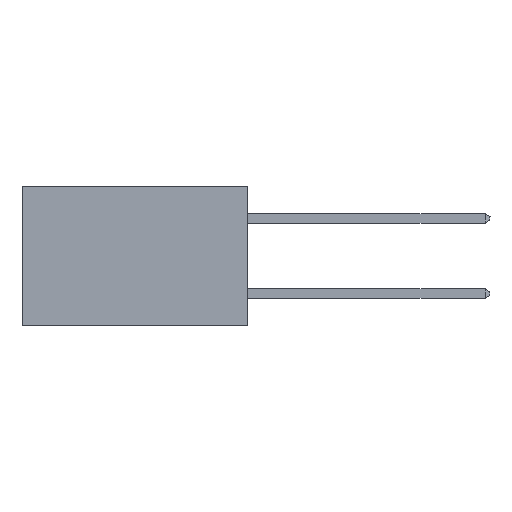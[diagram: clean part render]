
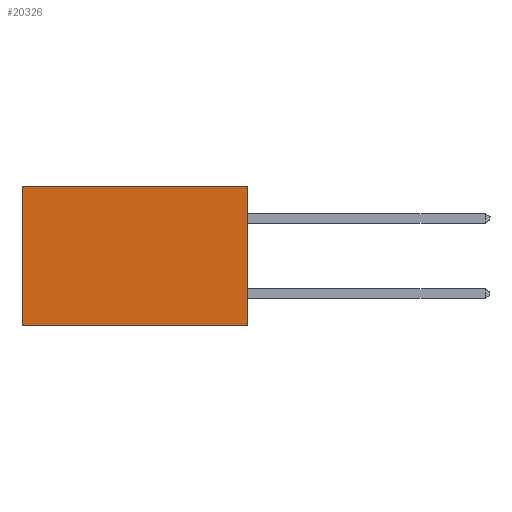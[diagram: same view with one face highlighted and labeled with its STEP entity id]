
A CAD part, left-side view. The second image highlights one B-rep face of the part: STEP entity #20326.
In plain terms, the highlighted planar face has unit normal (-1, 0, 0).
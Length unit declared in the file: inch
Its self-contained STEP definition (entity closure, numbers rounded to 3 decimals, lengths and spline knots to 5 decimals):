
#778 = LINE ( 'NONE', #7036, #1681 ) ;
#897 = FACE_OUTER_BOUND ( 'NONE', #9517, .T. ) ;
#1343 = LINE ( 'NONE', #14374, #9402 ) ;
#1681 = VECTOR ( 'NONE', #18409, 39.37008 ) ;
#2410 = VERTEX_POINT ( 'NONE', #12059 ) ;
#2424 = EDGE_CURVE ( 'NONE', #2410, #15097, #778, .T. ) ;
#2545 = VECTOR ( 'NONE', #6115, 39.37008 ) ;
#2762 = DIRECTION ( 'NONE',  ( 1., 0., 0. ) ) ;
#3389 = DIRECTION ( 'NONE',  ( 0., 1., 0. ) ) ;
#4240 = DIRECTION ( 'NONE',  ( 0., 0., -1. ) ) ;
#4374 = AXIS2_PLACEMENT_3D ( 'NONE', #18531, #2762, #4240 ) ;
#4376 = EDGE_CURVE ( 'NONE', #11083, #17826, #17289, .T. ) ;
#6115 = DIRECTION ( 'NONE',  ( 0., 0., -1. ) ) ;
#7036 = CARTESIAN_POINT ( 'NONE',  ( 0.2615, 0., 0. ) ) ;
#7144 = PLANE ( 'NONE',  #4374 ) ;
#7705 = DIRECTION ( 'NONE',  ( 0., 0., -1. ) ) ;
#8382 = ORIENTED_EDGE ( 'NONE', *, *, #13181, .T. ) ;
#8955 = EDGE_CURVE ( 'NONE', #2410, #11083, #1343, .T. ) ;
#9402 = VECTOR ( 'NONE', #7705, 39.37008 ) ;
#9517 = EDGE_LOOP ( 'NONE', ( #8382, #13086, #11619, #13781 ) ) ;
#9536 = LINE ( 'NONE', #15905, #2545 ) ;
#9650 = CARTESIAN_POINT ( 'NONE',  ( 0.2615, 0., -0.37 ) ) ;
#11083 = VERTEX_POINT ( 'NONE', #15057 ) ;
#11619 = ORIENTED_EDGE ( 'NONE', *, *, #8955, .F. ) ;
#12059 = CARTESIAN_POINT ( 'NONE',  ( 0.2615, 0., 0. ) ) ;
#12960 = CARTESIAN_POINT ( 'NONE',  ( 0.2615, 0.6, 0. ) ) ;
#13086 = ORIENTED_EDGE ( 'NONE', *, *, #4376, .F. ) ;
#13181 = EDGE_CURVE ( 'NONE', #15097, #17826, #9536, .T. ) ;
#13273 = VECTOR ( 'NONE', #3389, 39.37008 ) ;
#13781 = ORIENTED_EDGE ( 'NONE', *, *, #2424, .T. ) ;
#14374 = CARTESIAN_POINT ( 'NONE',  ( 0.2615, 0., -0.37 ) ) ;
#15057 = CARTESIAN_POINT ( 'NONE',  ( 0.2615, 0., -0.37 ) ) ;
#15097 = VERTEX_POINT ( 'NONE', #12960 ) ;
#15905 = CARTESIAN_POINT ( 'NONE',  ( 0.2615, 0.6, -0.37 ) ) ;
#17289 = LINE ( 'NONE', #9650, #13273 ) ;
#17665 = CARTESIAN_POINT ( 'NONE',  ( 0.2615, 0.6, -0.37 ) ) ;
#17826 = VERTEX_POINT ( 'NONE', #17665 ) ;
#18409 = DIRECTION ( 'NONE',  ( 0., 1., 0. ) ) ;
#18531 = CARTESIAN_POINT ( 'NONE',  ( 0.2615, 0., -0.37 ) ) ;
#20326 = ADVANCED_FACE ( 'NONE', ( #897 ), #7144, .F. ) ;
